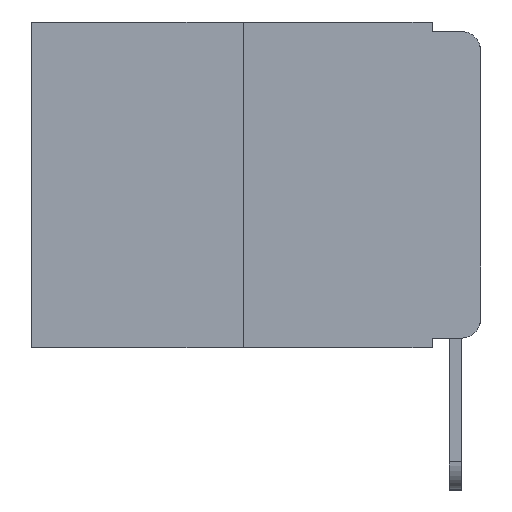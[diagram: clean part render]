
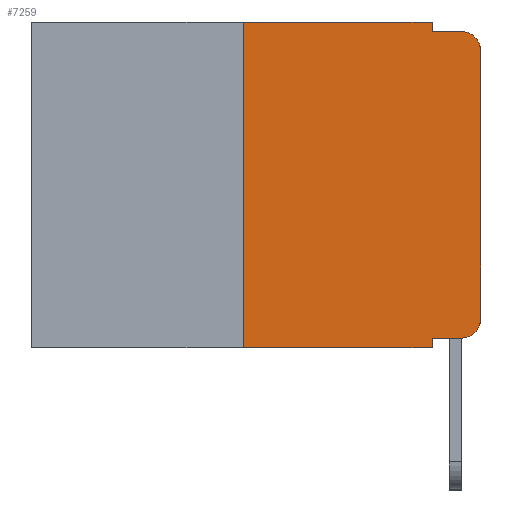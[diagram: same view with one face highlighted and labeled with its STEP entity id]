
A CAD part, left-side view. The second image highlights one B-rep face of the part: STEP entity #7259.
In plain terms, the highlighted planar face has unit normal (-1, 0, 0).
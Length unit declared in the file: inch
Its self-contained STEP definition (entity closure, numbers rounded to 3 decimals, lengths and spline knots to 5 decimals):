
#1037 = DIRECTION ( 'NONE',  ( 0., -1., 0. ) ) ;
#1453 = CARTESIAN_POINT ( 'NONE',  ( 0., 0., 0. ) ) ;
#1936 = DIRECTION ( 'NONE',  ( 0., -1., 0. ) ) ;
#1973 = VERTEX_POINT ( 'NONE', #6320 ) ;
#2007 = CARTESIAN_POINT ( 'NONE',  ( 0., 0.02, -0.03 ) ) ;
#2171 = CARTESIAN_POINT ( 'NONE',  ( 0., 0., -0.03 ) ) ;
#2356 = CARTESIAN_POINT ( 'NONE',  ( 0., 0.051, 0. ) ) ;
#2422 = VECTOR ( 'NONE', #22016, 39.37008 ) ;
#2489 = VERTEX_POINT ( 'NONE', #2356 ) ;
#3174 = ORIENTED_EDGE ( 'NONE', *, *, #16644, .T. ) ;
#3264 = VERTEX_POINT ( 'NONE', #25019 ) ;
#3529 = VERTEX_POINT ( 'NONE', #11891 ) ;
#3587 = VECTOR ( 'NONE', #10365, 39.37008 ) ;
#4152 = DIRECTION ( 'NONE',  ( 0., 0., -1. ) ) ;
#4297 = ORIENTED_EDGE ( 'NONE', *, *, #18427, .T. ) ;
#4378 = CARTESIAN_POINT ( 'NONE',  ( 0., 0.051, 0. ) ) ;
#4650 = CARTESIAN_POINT ( 'NONE',  ( 0., 0.02, -0.313 ) ) ;
#4765 = CARTESIAN_POINT ( 'NONE',  ( 0., 0.051, -0.333 ) ) ;
#4839 = ORIENTED_EDGE ( 'NONE', *, *, #9796, .F. ) ;
#5228 = ORIENTED_EDGE ( 'NONE', *, *, #5556, .F. ) ;
#5244 = EDGE_CURVE ( 'NONE', #7003, #12413, #23523, .T. ) ;
#5515 = ORIENTED_EDGE ( 'NONE', *, *, #19606, .F. ) ;
#5556 = EDGE_CURVE ( 'NONE', #2489, #3264, #22589, .T. ) ;
#5672 = VECTOR ( 'NONE', #10063, 39.37008 ) ;
#5788 = DIRECTION ( 'NONE',  ( 0., 0., 1. ) ) ;
#6204 = ORIENTED_EDGE ( 'NONE', *, *, #12953, .F. ) ;
#6320 = CARTESIAN_POINT ( 'NONE',  ( 0., 0.02, -0.01 ) ) ;
#6351 = LINE ( 'NONE', #22197, #5672 ) ;
#6827 = DIRECTION ( 'NONE',  ( 0., 0., -1. ) ) ;
#7003 = VERTEX_POINT ( 'NONE', #4765 ) ;
#7170 = ORIENTED_EDGE ( 'NONE', *, *, #17799, .T. ) ;
#7259 = ADVANCED_FACE ( 'NONE', ( #21599 ), #21805, .F. ) ;
#7693 = AXIS2_PLACEMENT_3D ( 'NONE', #17787, #25687, #13862 ) ;
#8125 = LINE ( 'NONE', #1453, #2422 ) ;
#8222 = ORIENTED_EDGE ( 'NONE', *, *, #22996, .F. ) ;
#8326 = CARTESIAN_POINT ( 'NONE',  ( 0., 0.473, 0. ) ) ;
#8671 = ORIENTED_EDGE ( 'NONE', *, *, #5244, .T. ) ;
#9548 = ORIENTED_EDGE ( 'NONE', *, *, #13942, .T. ) ;
#9761 = LINE ( 'NONE', #18018, #25656 ) ;
#9796 = EDGE_CURVE ( 'NONE', #3264, #1973, #6351, .T. ) ;
#9872 = LINE ( 'NONE', #8326, #3587 ) ;
#10063 = DIRECTION ( 'NONE',  ( 0., -1., 0. ) ) ;
#10186 = CARTESIAN_POINT ( 'NONE',  ( 0., 0.02, -0.333 ) ) ;
#10269 = VERTEX_POINT ( 'NONE', #21750 ) ;
#10365 = DIRECTION ( 'NONE',  ( 0., -1., 0. ) ) ;
#11467 = AXIS2_PLACEMENT_3D ( 'NONE', #2007, #16524, #4152 ) ;
#11516 = VECTOR ( 'NONE', #24681, 39.37008 ) ;
#11891 = CARTESIAN_POINT ( 'NONE',  ( 0., 0.051, -0.343 ) ) ;
#11929 = VERTEX_POINT ( 'NONE', #2171 ) ;
#11950 = VECTOR ( 'NONE', #22561, 39.37008 ) ;
#12413 = VERTEX_POINT ( 'NONE', #10186 ) ;
#12918 = VECTOR ( 'NONE', #1037, 39.37008 ) ;
#12953 = EDGE_CURVE ( 'NONE', #14631, #10269, #9761, .T. ) ;
#13862 = DIRECTION ( 'NONE',  ( 0., 0., -1. ) ) ;
#13942 = EDGE_CURVE ( 'NONE', #12413, #16043, #18524, .T. ) ;
#14539 = EDGE_LOOP ( 'NONE', ( #3174, #4297, #4839, #5228, #5515, #6204, #7170, #8222, #8671, #9548 ) ) ;
#14631 = VERTEX_POINT ( 'NONE', #17130 ) ;
#16043 = VERTEX_POINT ( 'NONE', #21618 ) ;
#16524 = DIRECTION ( 'NONE',  ( -1., 0., 0. ) ) ;
#16620 = LINE ( 'NONE', #24328, #21338 ) ;
#16644 = EDGE_CURVE ( 'NONE', #16043, #11929, #8125, .T. ) ;
#17130 = CARTESIAN_POINT ( 'NONE',  ( 0., 0.25, -0.343 ) ) ;
#17787 = CARTESIAN_POINT ( 'NONE',  ( 0., 0.473, 0. ) ) ;
#17799 = EDGE_CURVE ( 'NONE', #14631, #3529, #16620, .T. ) ;
#18018 = CARTESIAN_POINT ( 'NONE',  ( 0., 0.25, 0. ) ) ;
#18427 = EDGE_CURVE ( 'NONE', #11929, #1973, #22214, .T. ) ;
#18524 = CIRCLE ( 'NONE', #26028, 0.02 ) ;
#19002 = DIRECTION ( 'NONE',  ( -1., 0., 0. ) ) ;
#19606 = EDGE_CURVE ( 'NONE', #10269, #2489, #9872, .T. ) ;
#21338 = VECTOR ( 'NONE', #1936, 39.37008 ) ;
#21561 = LINE ( 'NONE', #4378, #11516 ) ;
#21599 = FACE_OUTER_BOUND ( 'NONE', #14539, .T. ) ;
#21618 = CARTESIAN_POINT ( 'NONE',  ( 0., 0., -0.313 ) ) ;
#21750 = CARTESIAN_POINT ( 'NONE',  ( 0., 0.25, 0. ) ) ;
#21805 = PLANE ( 'NONE',  #7693 ) ;
#22016 = DIRECTION ( 'NONE',  ( 0., 0., 1. ) ) ;
#22197 = CARTESIAN_POINT ( 'NONE',  ( 0., 0.051, -0.01 ) ) ;
#22214 = CIRCLE ( 'NONE', #11467, 0.02 ) ;
#22561 = DIRECTION ( 'NONE',  ( 0., 0., -1. ) ) ;
#22589 = LINE ( 'NONE', #24498, #11950 ) ;
#22996 = EDGE_CURVE ( 'NONE', #7003, #3529, #21561, .T. ) ;
#23523 = LINE ( 'NONE', #25444, #12918 ) ;
#24328 = CARTESIAN_POINT ( 'NONE',  ( 0., 0.473, -0.343 ) ) ;
#24498 = CARTESIAN_POINT ( 'NONE',  ( 0., 0.051, 0. ) ) ;
#24681 = DIRECTION ( 'NONE',  ( 0., 0., -1. ) ) ;
#25019 = CARTESIAN_POINT ( 'NONE',  ( 0., 0.051, -0.01 ) ) ;
#25444 = CARTESIAN_POINT ( 'NONE',  ( 0., 0.051, -0.333 ) ) ;
#25656 = VECTOR ( 'NONE', #5788, 39.37008 ) ;
#25687 = DIRECTION ( 'NONE',  ( 1., 0., 0. ) ) ;
#26028 = AXIS2_PLACEMENT_3D ( 'NONE', #4650, #19002, #6827 ) ;
